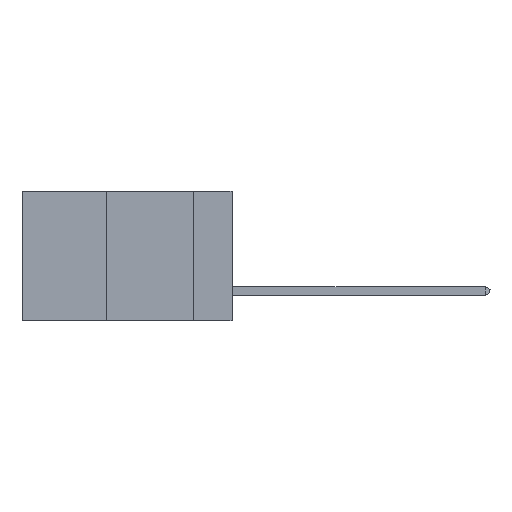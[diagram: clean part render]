
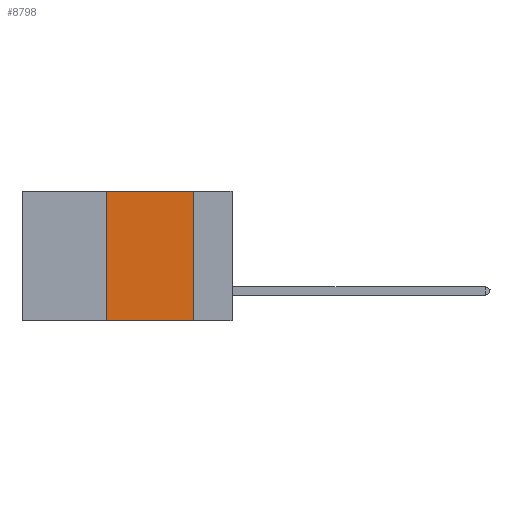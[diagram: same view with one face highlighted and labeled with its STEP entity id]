
A CAD part, left-side view. The second image highlights one B-rep face of the part: STEP entity #8798.
In plain terms, the highlighted planar face has unit normal (-1, 0, 0).
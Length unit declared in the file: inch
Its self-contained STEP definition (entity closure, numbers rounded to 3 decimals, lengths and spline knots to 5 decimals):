
#379 = ORIENTED_EDGE ( 'NONE', *, *, #5467, .F. ) ;
#876 = AXIS2_PLACEMENT_3D ( 'NONE', #4788, #6049, #7198 ) ;
#2537 = VECTOR ( 'NONE', #3478, 39.37008 ) ;
#2972 = VERTEX_POINT ( 'NONE', #11204 ) ;
#2977 = VERTEX_POINT ( 'NONE', #6725 ) ;
#3046 = VECTOR ( 'NONE', #4507, 39.37008 ) ;
#3442 = LINE ( 'NONE', #9500, #3046 ) ;
#3478 = DIRECTION ( 'NONE',  ( 0., -1., 0. ) ) ;
#4410 = LINE ( 'NONE', #6256, #5749 ) ;
#4507 = DIRECTION ( 'NONE',  ( 0., 0., 1. ) ) ;
#4788 = CARTESIAN_POINT ( 'NONE',  ( 0., 0.6, 0. ) ) ;
#4800 = CARTESIAN_POINT ( 'NONE',  ( 0., 0.11, 0. ) ) ;
#4899 = EDGE_LOOP ( 'NONE', ( #13639, #379, #16040, #11982 ) ) ;
#4983 = VECTOR ( 'NONE', #13019, 39.37008 ) ;
#5467 = EDGE_CURVE ( 'NONE', #2972, #6085, #10078, .T. ) ;
#5749 = VECTOR ( 'NONE', #13881, 39.37008 ) ;
#5937 = CARTESIAN_POINT ( 'NONE',  ( 0., 0.6, 0. ) ) ;
#6049 = DIRECTION ( 'NONE',  ( 1., 0., 0. ) ) ;
#6085 = VERTEX_POINT ( 'NONE', #4800 ) ;
#6256 = CARTESIAN_POINT ( 'NONE',  ( 0., 0.6, -0.37 ) ) ;
#6725 = CARTESIAN_POINT ( 'NONE',  ( 0., 0.36, -0.37 ) ) ;
#7058 = EDGE_CURVE ( 'NONE', #6085, #11220, #10596, .T. ) ;
#7198 = DIRECTION ( 'NONE',  ( 0., 0., -1. ) ) ;
#7391 = EDGE_CURVE ( 'NONE', #2977, #11220, #4410, .T. ) ;
#7691 = FACE_OUTER_BOUND ( 'NONE', #4899, .T. ) ;
#8492 = PLANE ( 'NONE',  #876 ) ;
#8798 = ADVANCED_FACE ( 'NONE', ( #7691 ), #8492, .F. ) ;
#8868 = CARTESIAN_POINT ( 'NONE',  ( 0., 0.11, -0.37 ) ) ;
#9447 = CARTESIAN_POINT ( 'NONE',  ( 0., 0.11, 0. ) ) ;
#9500 = CARTESIAN_POINT ( 'NONE',  ( 0., 0.36, 0. ) ) ;
#10078 = LINE ( 'NONE', #5937, #2537 ) ;
#10596 = LINE ( 'NONE', #9447, #4983 ) ;
#11204 = CARTESIAN_POINT ( 'NONE',  ( 0., 0.36, 0. ) ) ;
#11220 = VERTEX_POINT ( 'NONE', #8868 ) ;
#11982 = ORIENTED_EDGE ( 'NONE', *, *, #7391, .T. ) ;
#13019 = DIRECTION ( 'NONE',  ( 0., 0., -1. ) ) ;
#13639 = ORIENTED_EDGE ( 'NONE', *, *, #7058, .F. ) ;
#13881 = DIRECTION ( 'NONE',  ( 0., -1., 0. ) ) ;
#14051 = EDGE_CURVE ( 'NONE', #2977, #2972, #3442, .T. ) ;
#16040 = ORIENTED_EDGE ( 'NONE', *, *, #14051, .F. ) ;
